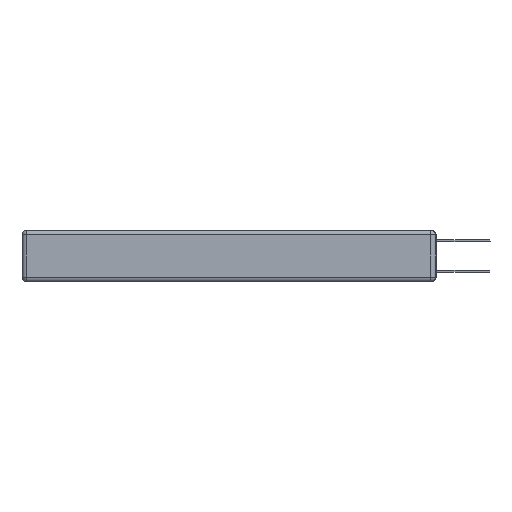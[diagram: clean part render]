
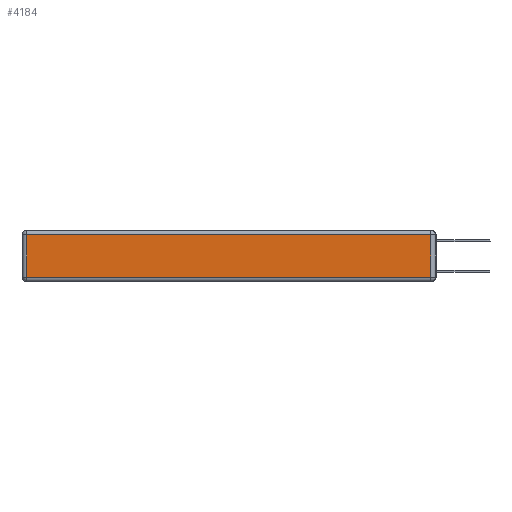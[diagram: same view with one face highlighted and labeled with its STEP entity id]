
A CAD part, left-side view. The second image highlights one B-rep face of the part: STEP entity #4184.
In plain terms, the highlighted planar face has unit normal (-1, 0, 0).
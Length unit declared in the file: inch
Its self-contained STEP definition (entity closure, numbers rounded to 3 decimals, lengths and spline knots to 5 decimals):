
#2810 = CARTESIAN_POINT ( 'NONE',  ( 0., 0.03, -0.313 ) ) ;
#3080 = LINE ( 'NONE', #14315, #13400 ) ;
#3200 = LINE ( 'NONE', #9434, #14823 ) ;
#3873 = AXIS2_PLACEMENT_3D ( 'NONE', #4580, #20580, #14218 ) ;
#4184 = ADVANCED_FACE ( 'NONE', ( #15809 ), #9642, .T. ) ;
#4253 = ORIENTED_EDGE ( 'NONE', *, *, #9338, .T. ) ;
#4580 = CARTESIAN_POINT ( 'NONE',  ( 0., 0., -0.343 ) ) ;
#4859 = DIRECTION ( 'NONE',  ( 0., 0., -1. ) ) ;
#5562 = VERTEX_POINT ( 'NONE', #5640 ) ;
#5605 = EDGE_CURVE ( 'NONE', #10604, #10110, #3080, .T. ) ;
#5640 = CARTESIAN_POINT ( 'NONE',  ( 0., 2.72, -0.03 ) ) ;
#5820 = LINE ( 'NONE', #15265, #17039 ) ;
#5923 = ORIENTED_EDGE ( 'NONE', *, *, #5605, .T. ) ;
#7311 = DIRECTION ( 'NONE',  ( 0., 1., 0. ) ) ;
#7939 = DIRECTION ( 'NONE',  ( 0., -1., 0. ) ) ;
#7954 = DIRECTION ( 'NONE',  ( 0., 0., 1. ) ) ;
#9032 = CARTESIAN_POINT ( 'NONE',  ( 0., 2.72, -0.313 ) ) ;
#9338 = EDGE_CURVE ( 'NONE', #10110, #17668, #3200, .T. ) ;
#9434 = CARTESIAN_POINT ( 'NONE',  ( 0., 0.03, -0.343 ) ) ;
#9642 = PLANE ( 'NONE',  #3873 ) ;
#10110 = VERTEX_POINT ( 'NONE', #2810 ) ;
#10432 = EDGE_LOOP ( 'NONE', ( #5923, #4253, #19838, #10895 ) ) ;
#10599 = VECTOR ( 'NONE', #4859, 39.37008 ) ;
#10604 = VERTEX_POINT ( 'NONE', #9032 ) ;
#10895 = ORIENTED_EDGE ( 'NONE', *, *, #20483, .T. ) ;
#12451 = CARTESIAN_POINT ( 'NONE',  ( 0., 0.03, -0.03 ) ) ;
#13400 = VECTOR ( 'NONE', #7939, 39.37008 ) ;
#14218 = DIRECTION ( 'NONE',  ( 0., 0., 1. ) ) ;
#14315 = CARTESIAN_POINT ( 'NONE',  ( 0., 0., -0.313 ) ) ;
#14823 = VECTOR ( 'NONE', #7954, 39.37008 ) ;
#15265 = CARTESIAN_POINT ( 'NONE',  ( 0., 2.75, -0.03 ) ) ;
#15809 = FACE_OUTER_BOUND ( 'NONE', #10432, .T. ) ;
#15990 = LINE ( 'NONE', #17480, #10599 ) ;
#17039 = VECTOR ( 'NONE', #7311, 39.37008 ) ;
#17480 = CARTESIAN_POINT ( 'NONE',  ( 0., 2.72, -0.343 ) ) ;
#17668 = VERTEX_POINT ( 'NONE', #12451 ) ;
#19112 = EDGE_CURVE ( 'NONE', #17668, #5562, #5820, .T. ) ;
#19838 = ORIENTED_EDGE ( 'NONE', *, *, #19112, .T. ) ;
#20483 = EDGE_CURVE ( 'NONE', #5562, #10604, #15990, .T. ) ;
#20580 = DIRECTION ( 'NONE',  ( -1., 0., 0. ) ) ;
